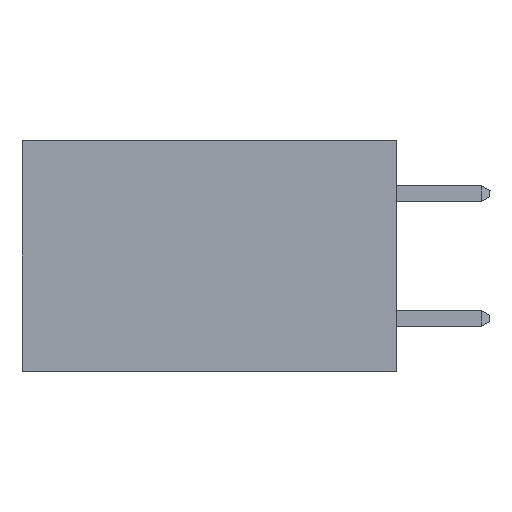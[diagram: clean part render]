
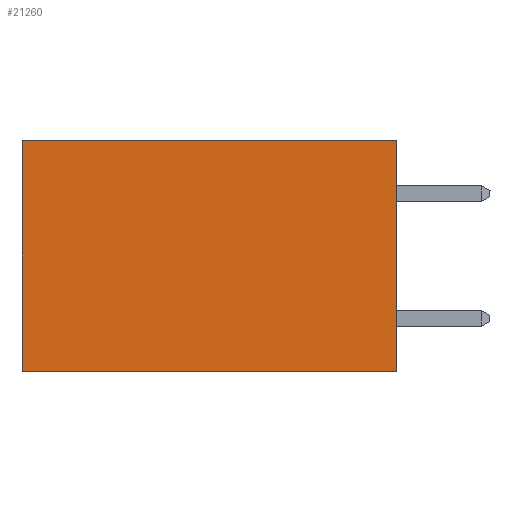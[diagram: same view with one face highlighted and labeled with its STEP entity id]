
A CAD part, left-side view. The second image highlights one B-rep face of the part: STEP entity #21260.
In plain terms, the highlighted planar face has unit normal (-1, 0, 0).
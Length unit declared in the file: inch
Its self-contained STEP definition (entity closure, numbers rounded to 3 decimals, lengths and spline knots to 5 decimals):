
#138 = VERTEX_POINT ( 'NONE', #2712 ) ;
#290 = ORIENTED_EDGE ( 'NONE', *, *, #7462, .T. ) ;
#902 = VERTEX_POINT ( 'NONE', #9199 ) ;
#1552 = DIRECTION ( 'NONE',  ( 0., 0., -1. ) ) ;
#1561 = DIRECTION ( 'NONE',  ( 0., 1., 0. ) ) ;
#2139 = EDGE_CURVE ( 'NONE', #902, #4360, #19544, .T. ) ;
#2652 = LINE ( 'NONE', #12177, #10988 ) ;
#2712 = CARTESIAN_POINT ( 'NONE',  ( 0.298, 0., -0.37 ) ) ;
#2825 = PLANE ( 'NONE',  #17334 ) ;
#3051 = EDGE_CURVE ( 'NONE', #902, #138, #9628, .T. ) ;
#4360 = VERTEX_POINT ( 'NONE', #14527 ) ;
#5296 = ORIENTED_EDGE ( 'NONE', *, *, #11858, .F. ) ;
#6064 = EDGE_LOOP ( 'NONE', ( #290, #5296, #14534, #20196 ) ) ;
#6901 = CARTESIAN_POINT ( 'NONE',  ( 0.298, 0.6, 0. ) ) ;
#6929 = DIRECTION ( 'NONE',  ( 0., 0., -1. ) ) ;
#7462 = EDGE_CURVE ( 'NONE', #4360, #18425, #17941, .T. ) ;
#8104 = CARTESIAN_POINT ( 'NONE',  ( 0.298, 0., 0. ) ) ;
#8277 = DIRECTION ( 'NONE',  ( 1., 0., 0. ) ) ;
#8561 = VECTOR ( 'NONE', #1552, 39.37008 ) ;
#8828 = CARTESIAN_POINT ( 'NONE',  ( 0.298, 0.6, -0.37 ) ) ;
#9090 = VECTOR ( 'NONE', #6929, 39.37008 ) ;
#9199 = CARTESIAN_POINT ( 'NONE',  ( 0.298, 0., 0. ) ) ;
#9628 = LINE ( 'NONE', #15172, #9090 ) ;
#9675 = VECTOR ( 'NONE', #16436, 39.37008 ) ;
#10988 = VECTOR ( 'NONE', #1561, 39.37008 ) ;
#11858 = EDGE_CURVE ( 'NONE', #138, #18425, #2652, .T. ) ;
#12177 = CARTESIAN_POINT ( 'NONE',  ( 0.298, 0., -0.37 ) ) ;
#14527 = CARTESIAN_POINT ( 'NONE',  ( 0.298, 0.6, 0. ) ) ;
#14534 = ORIENTED_EDGE ( 'NONE', *, *, #3051, .F. ) ;
#15172 = CARTESIAN_POINT ( 'NONE',  ( 0.298, 0., 0. ) ) ;
#16436 = DIRECTION ( 'NONE',  ( 0., 1., 0. ) ) ;
#17334 = AXIS2_PLACEMENT_3D ( 'NONE', #18799, #8277, #20484 ) ;
#17941 = LINE ( 'NONE', #6901, #8561 ) ;
#18044 = FACE_OUTER_BOUND ( 'NONE', #6064, .T. ) ;
#18425 = VERTEX_POINT ( 'NONE', #8828 ) ;
#18799 = CARTESIAN_POINT ( 'NONE',  ( 0.298, 0., 0. ) ) ;
#19544 = LINE ( 'NONE', #8104, #9675 ) ;
#20196 = ORIENTED_EDGE ( 'NONE', *, *, #2139, .T. ) ;
#20484 = DIRECTION ( 'NONE',  ( 0., 0., -1. ) ) ;
#21260 = ADVANCED_FACE ( 'NONE', ( #18044 ), #2825, .F. ) ;
